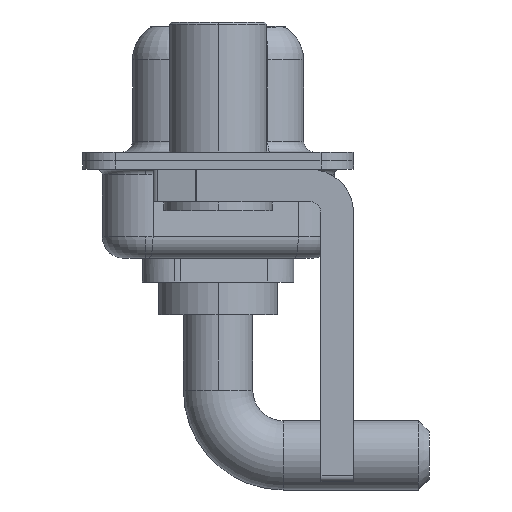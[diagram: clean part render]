
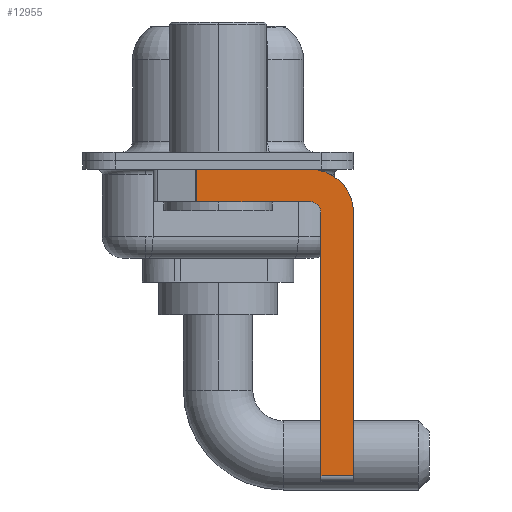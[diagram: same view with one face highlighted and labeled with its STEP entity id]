
A CAD part, left-side view. The second image highlights one B-rep face of the part: STEP entity #12955.
In plain terms, the highlighted planar face has unit normal (-1, 0, 0).
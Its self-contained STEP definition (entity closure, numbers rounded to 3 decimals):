
#294 = EDGE_CURVE ( 'NONE', #11547, #4568, #1118, .T. ) ;
#642 = EDGE_CURVE ( 'NONE', #6788, #1507, #12465, .T. ) ;
#735 = CARTESIAN_POINT ( 'NONE',  ( -2.9, 0.978, -1.9 ) ) ;
#965 = AXIS2_PLACEMENT_3D ( 'NONE', #6583, #1802, #13824 ) ;
#1094 = VECTOR ( 'NONE', #6229, 1000. ) ;
#1118 = LINE ( 'NONE', #11597, #12713 ) ;
#1146 = CARTESIAN_POINT ( 'NONE',  ( -2.9, 0.978, -0.4 ) ) ;
#1210 = CIRCLE ( 'NONE', #965, 0.5 ) ;
#1229 = DIRECTION ( 'NONE',  ( 1., 0., 0. ) ) ;
#1233 = CARTESIAN_POINT ( 'NONE',  ( -2.9, -6.25, -2.4 ) ) ;
#1276 = ORIENTED_EDGE ( 'NONE', *, *, #5593, .F. ) ;
#1494 = LINE ( 'NONE', #3883, #7137 ) ;
#1507 = VERTEX_POINT ( 'NONE', #1233 ) ;
#1802 = DIRECTION ( 'NONE',  ( -1., 0., 0. ) ) ;
#2257 = ORIENTED_EDGE ( 'NONE', *, *, #3157, .F. ) ;
#2426 = EDGE_LOOP ( 'NONE', ( #1276, #7946, #12575, #2257, #6026, #9388, #7676, #11555 ) ) ;
#3045 = CARTESIAN_POINT ( 'NONE',  ( -2.9, -4.25, -2.4 ) ) ;
#3118 = VECTOR ( 'NONE', #4255, 1000. ) ;
#3157 = EDGE_CURVE ( 'NONE', #7024, #11547, #1210, .T. ) ;
#3184 = CARTESIAN_POINT ( 'NONE',  ( -2.9, -6.25, -14.55 ) ) ;
#3708 = VECTOR ( 'NONE', #9741, 1000. ) ;
#3711 = LINE ( 'NONE', #9808, #3708 ) ;
#3883 = CARTESIAN_POINT ( 'NONE',  ( -2.9, 3., -0.4 ) ) ;
#4255 = DIRECTION ( 'NONE',  ( 0., 0., -1. ) ) ;
#4568 = VERTEX_POINT ( 'NONE', #735 ) ;
#5062 = CARTESIAN_POINT ( 'NONE',  ( -2.9, -4.75, -14.8 ) ) ;
#5359 = CARTESIAN_POINT ( 'NONE',  ( -2.9, -4.25, -0.4 ) ) ;
#5593 = EDGE_CURVE ( 'NONE', #10075, #6788, #1494, .T. ) ;
#5648 = DIRECTION ( 'NONE',  ( 1., 0., 0. ) ) ;
#6026 = ORIENTED_EDGE ( 'NONE', *, *, #10602, .F. ) ;
#6106 = EDGE_CURVE ( 'NONE', #1507, #13392, #3711, .T. ) ;
#6229 = DIRECTION ( 'NONE',  ( 0., 0., 1. ) ) ;
#6583 = CARTESIAN_POINT ( 'NONE',  ( -2.9, -4.25, -2.4 ) ) ;
#6639 = LINE ( 'NONE', #14657, #3118 ) ;
#6788 = VERTEX_POINT ( 'NONE', #5359 ) ;
#6811 = AXIS2_PLACEMENT_3D ( 'NONE', #3045, #5648, #13528 ) ;
#6894 = CARTESIAN_POINT ( 'NONE',  ( -2.9, -4.75, -2.4 ) ) ;
#7024 = VERTEX_POINT ( 'NONE', #6894 ) ;
#7137 = VECTOR ( 'NONE', #7200, 1000. ) ;
#7200 = DIRECTION ( 'NONE',  ( 0., -1., 0. ) ) ;
#7393 = CARTESIAN_POINT ( 'NONE',  ( -2.9, -4.25, -1.9 ) ) ;
#7676 = ORIENTED_EDGE ( 'NONE', *, *, #6106, .F. ) ;
#7946 = ORIENTED_EDGE ( 'NONE', *, *, #14208, .T. ) ;
#8136 = DIRECTION ( 'NONE',  ( 0., 1., 0. ) ) ;
#8492 = PLANE ( 'NONE',  #12272 ) ;
#8875 = CARTESIAN_POINT ( 'NONE',  ( -2.9, -4.75, -14.55 ) ) ;
#9388 = ORIENTED_EDGE ( 'NONE', *, *, #14486, .T. ) ;
#9654 = DIRECTION ( 'NONE',  ( 0., 0., -1. ) ) ;
#9734 = FACE_OUTER_BOUND ( 'NONE', #2426, .T. ) ;
#9741 = DIRECTION ( 'NONE',  ( 0., 0., -1. ) ) ;
#9808 = CARTESIAN_POINT ( 'NONE',  ( -2.9, -6.25, -2.4 ) ) ;
#10044 = LINE ( 'NONE', #14592, #13199 ) ;
#10075 = VERTEX_POINT ( 'NONE', #1146 ) ;
#10602 = EDGE_CURVE ( 'NONE', #14187, #7024, #10841, .T. ) ;
#10841 = LINE ( 'NONE', #5062, #1094 ) ;
#11547 = VERTEX_POINT ( 'NONE', #7393 ) ;
#11555 = ORIENTED_EDGE ( 'NONE', *, *, #642, .F. ) ;
#11597 = CARTESIAN_POINT ( 'NONE',  ( -2.9, -4.25, -1.9 ) ) ;
#12265 = DIRECTION ( 'NONE',  ( 0., -1., 0. ) ) ;
#12272 = AXIS2_PLACEMENT_3D ( 'NONE', #14120, #1229, #9654 ) ;
#12465 = CIRCLE ( 'NONE', #6811, 2. ) ;
#12575 = ORIENTED_EDGE ( 'NONE', *, *, #294, .F. ) ;
#12713 = VECTOR ( 'NONE', #8136, 1000. ) ;
#12955 = ADVANCED_FACE ( 'NONE', ( #9734 ), #8492, .F. ) ;
#13199 = VECTOR ( 'NONE', #12265, 1000. ) ;
#13392 = VERTEX_POINT ( 'NONE', #3184 ) ;
#13528 = DIRECTION ( 'NONE',  ( 0., 0., -1. ) ) ;
#13824 = DIRECTION ( 'NONE',  ( 0., 0., 1. ) ) ;
#14120 = CARTESIAN_POINT ( 'NONE',  ( -2.9, -4.25, -2.4 ) ) ;
#14187 = VERTEX_POINT ( 'NONE', #8875 ) ;
#14208 = EDGE_CURVE ( 'NONE', #10075, #4568, #6639, .T. ) ;
#14486 = EDGE_CURVE ( 'NONE', #14187, #13392, #10044, .T. ) ;
#14592 = CARTESIAN_POINT ( 'NONE',  ( -2.9, -4.25, -14.55 ) ) ;
#14657 = CARTESIAN_POINT ( 'NONE',  ( -2.9, 0.978, -1.9 ) ) ;
